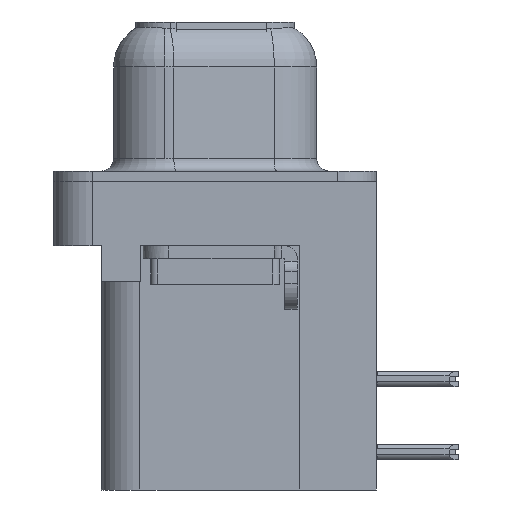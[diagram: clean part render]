
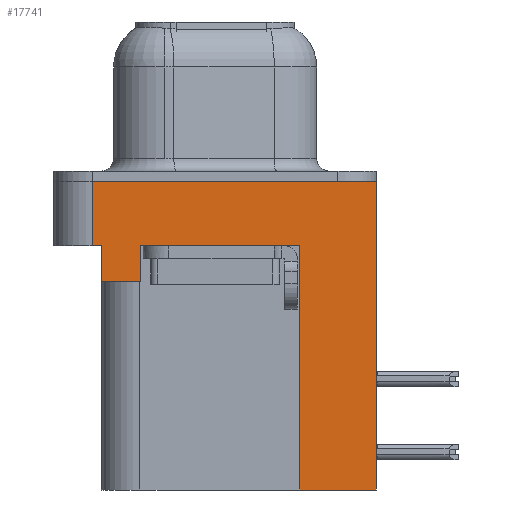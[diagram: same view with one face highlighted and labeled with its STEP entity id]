
A CAD part, left-side view. The second image highlights one B-rep face of the part: STEP entity #17741.
In plain terms, the highlighted planar face has unit normal (-1, 0, 0).
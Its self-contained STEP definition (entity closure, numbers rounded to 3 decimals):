
#163 = CARTESIAN_POINT ( 'NONE',  ( -2.935, 2.895, -2.5 ) ) ;
#231 = LINE ( 'NONE', #9095, #14035 ) ;
#261 = ORIENTED_EDGE ( 'NONE', *, *, #1286, .T. ) ;
#432 = EDGE_CURVE ( 'NONE', #10324, #10980, #8036, .T. ) ;
#763 = ORIENTED_EDGE ( 'NONE', *, *, #5312, .T. ) ;
#1286 = EDGE_CURVE ( 'NONE', #17852, #18541, #2996, .T. ) ;
#1694 = DIRECTION ( 'NONE',  ( 0., 0., 1. ) ) ;
#2229 = VERTEX_POINT ( 'NONE', #19236 ) ;
#2568 = CARTESIAN_POINT ( 'NONE',  ( -2.935, 4.775, 0. ) ) ;
#2828 = VERTEX_POINT ( 'NONE', #18016 ) ;
#2996 = LINE ( 'NONE', #22229, #3010 ) ;
#3010 = VECTOR ( 'NONE', #22239, 1000. ) ;
#3495 = VERTEX_POINT ( 'NONE', #21514 ) ;
#3610 = DIRECTION ( 'NONE',  ( -1., 0., 0. ) ) ;
#4358 = DIRECTION ( 'NONE',  ( 0., -1., 0. ) ) ;
#4513 = LINE ( 'NONE', #17504, #10113 ) ;
#4876 = AXIS2_PLACEMENT_3D ( 'NONE', #16547, #3610, #16730 ) ;
#5000 = EDGE_LOOP ( 'NONE', ( #15739, #18843, #763, #9911, #19225, #8807, #261, #12302, #21133, #6535 ) ) ;
#5312 = EDGE_CURVE ( 'NONE', #10324, #12337, #13228, .T. ) ;
#5410 = CARTESIAN_POINT ( 'NONE',  ( -2.935, -6.275, -2.5 ) ) ;
#5756 = VECTOR ( 'NONE', #21363, 1000. ) ;
#6535 = ORIENTED_EDGE ( 'NONE', *, *, #13072, .T. ) ;
#6683 = LINE ( 'NONE', #18151, #21094 ) ;
#6767 = EDGE_CURVE ( 'NONE', #2229, #18541, #6683, .T. ) ;
#7385 = DIRECTION ( 'NONE',  ( 0., 0., 1. ) ) ;
#7464 = EDGE_CURVE ( 'NONE', #3495, #17852, #231, .T. ) ;
#7546 = LINE ( 'NONE', #22319, #17612 ) ;
#8036 = LINE ( 'NONE', #9586, #8086 ) ;
#8086 = VECTOR ( 'NONE', #19851, 1000. ) ;
#8174 = VECTOR ( 'NONE', #20206, 1000. ) ;
#8223 = DIRECTION ( 'NONE',  ( 0., 1., 0. ) ) ;
#8707 = DIRECTION ( 'NONE',  ( 0., 0., 1. ) ) ;
#8730 = CARTESIAN_POINT ( 'NONE',  ( -2.935, 4.425, -2.5 ) ) ;
#8807 = ORIENTED_EDGE ( 'NONE', *, *, #7464, .T. ) ;
#8873 = VECTOR ( 'NONE', #8223, 1000. ) ;
#9095 = CARTESIAN_POINT ( 'NONE',  ( -2.935, 2.895, -3.9 ) ) ;
#9278 = VERTEX_POINT ( 'NONE', #24228 ) ;
#9586 = CARTESIAN_POINT ( 'NONE',  ( -2.935, 4.775, -2.5 ) ) ;
#9749 = EDGE_CURVE ( 'NONE', #9278, #12337, #7546, .T. ) ;
#9817 = FACE_OUTER_BOUND ( 'NONE', #5000, .T. ) ;
#9911 = ORIENTED_EDGE ( 'NONE', *, *, #9749, .F. ) ;
#10113 = VECTOR ( 'NONE', #4358, 1000. ) ;
#10130 = CARTESIAN_POINT ( 'NONE',  ( -2.935, 4.425, -3.9 ) ) ;
#10163 = VECTOR ( 'NONE', #1694, 1000. ) ;
#10165 = CARTESIAN_POINT ( 'NONE',  ( -2.935, -3.295, -12. ) ) ;
#10324 = VERTEX_POINT ( 'NONE', #19173 ) ;
#10980 = VERTEX_POINT ( 'NONE', #2568 ) ;
#11963 = LINE ( 'NONE', #10130, #5756 ) ;
#12302 = ORIENTED_EDGE ( 'NONE', *, *, #6767, .F. ) ;
#12337 = VERTEX_POINT ( 'NONE', #8730 ) ;
#12963 = CARTESIAN_POINT ( 'NONE',  ( -2.935, -6.275, -12. ) ) ;
#13072 = EDGE_CURVE ( 'NONE', #18343, #2828, #20147, .T. ) ;
#13228 = LINE ( 'NONE', #5410, #8174 ) ;
#13880 = LINE ( 'NONE', #10165, #8873 ) ;
#14035 = VECTOR ( 'NONE', #8707, 1000. ) ;
#14819 = PLANE ( 'NONE',  #4876 ) ;
#15739 = ORIENTED_EDGE ( 'NONE', *, *, #17984, .F. ) ;
#16547 = CARTESIAN_POINT ( 'NONE',  ( -2.935, -6.275, -2.5 ) ) ;
#16730 = DIRECTION ( 'NONE',  ( 0., 0., 1. ) ) ;
#17504 = CARTESIAN_POINT ( 'NONE',  ( -2.935, -6.275, 0. ) ) ;
#17612 = VECTOR ( 'NONE', #7385, 1000. ) ;
#17651 = CARTESIAN_POINT ( 'NONE',  ( -2.935, -3.295, -2.5 ) ) ;
#17741 = ADVANCED_FACE ( 'NONE', ( #9817 ), #14819, .T. ) ;
#17852 = VERTEX_POINT ( 'NONE', #163 ) ;
#17984 = EDGE_CURVE ( 'NONE', #10980, #2828, #4513, .T. ) ;
#18016 = CARTESIAN_POINT ( 'NONE',  ( -2.935, -6.275, 0. ) ) ;
#18151 = CARTESIAN_POINT ( 'NONE',  ( -2.935, -3.295, -12. ) ) ;
#18343 = VERTEX_POINT ( 'NONE', #12963 ) ;
#18406 = DIRECTION ( 'NONE',  ( 0., 0., 1. ) ) ;
#18541 = VERTEX_POINT ( 'NONE', #17651 ) ;
#18547 = EDGE_CURVE ( 'NONE', #18343, #2229, #13880, .T. ) ;
#18843 = ORIENTED_EDGE ( 'NONE', *, *, #432, .F. ) ;
#19173 = CARTESIAN_POINT ( 'NONE',  ( -2.935, 4.775, -2.5 ) ) ;
#19225 = ORIENTED_EDGE ( 'NONE', *, *, #23331, .F. ) ;
#19236 = CARTESIAN_POINT ( 'NONE',  ( -2.935, -3.295, -12. ) ) ;
#19851 = DIRECTION ( 'NONE',  ( 0., 0., 1. ) ) ;
#20147 = LINE ( 'NONE', #24117, #10163 ) ;
#20206 = DIRECTION ( 'NONE',  ( 0., -1., 0. ) ) ;
#21094 = VECTOR ( 'NONE', #18406, 1000. ) ;
#21133 = ORIENTED_EDGE ( 'NONE', *, *, #18547, .F. ) ;
#21363 = DIRECTION ( 'NONE',  ( 0., 1., 0. ) ) ;
#21514 = CARTESIAN_POINT ( 'NONE',  ( -2.935, 2.895, -3.9 ) ) ;
#22229 = CARTESIAN_POINT ( 'NONE',  ( -2.935, -6.275, -2.5 ) ) ;
#22239 = DIRECTION ( 'NONE',  ( 0., -1., 0. ) ) ;
#22319 = CARTESIAN_POINT ( 'NONE',  ( -2.935, 4.425, -3.9 ) ) ;
#23331 = EDGE_CURVE ( 'NONE', #3495, #9278, #11963, .T. ) ;
#24117 = CARTESIAN_POINT ( 'NONE',  ( -2.935, -6.275, -2.5 ) ) ;
#24228 = CARTESIAN_POINT ( 'NONE',  ( -2.935, 4.425, -3.9 ) ) ;
